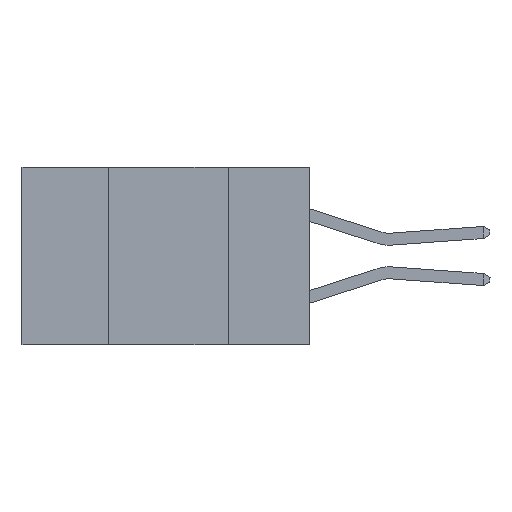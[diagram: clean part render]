
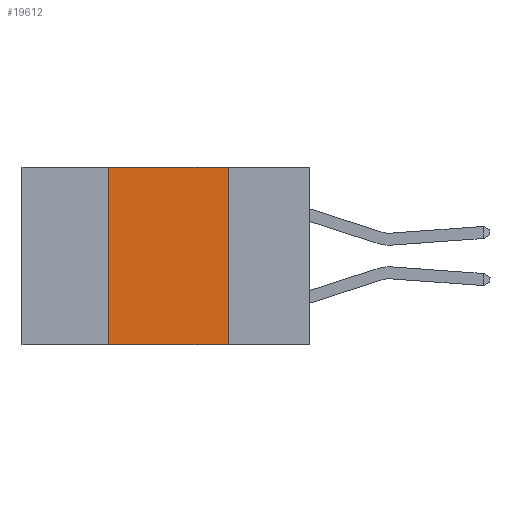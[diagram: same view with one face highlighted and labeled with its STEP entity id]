
A CAD part, left-side view. The second image highlights one B-rep face of the part: STEP entity #19612.
In plain terms, the highlighted planar face has unit normal (-1, 0, 0).
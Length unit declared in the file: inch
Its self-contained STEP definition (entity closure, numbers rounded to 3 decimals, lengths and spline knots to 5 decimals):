
#87 = EDGE_CURVE ( 'NONE', #4381, #3014, #8538, .T. ) ;
#420 = FACE_OUTER_BOUND ( 'NONE', #12172, .T. ) ;
#507 = CARTESIAN_POINT ( 'NONE',  ( 0., 0.42, 0. ) ) ;
#776 = LINE ( 'NONE', #15083, #2478 ) ;
#1242 = CARTESIAN_POINT ( 'NONE',  ( 0., 0.17, 0. ) ) ;
#1489 = CARTESIAN_POINT ( 'NONE',  ( 0., 0.6, 0. ) ) ;
#2449 = VERTEX_POINT ( 'NONE', #6908 ) ;
#2478 = VECTOR ( 'NONE', #12122, 39.37008 ) ;
#3014 = VERTEX_POINT ( 'NONE', #16948 ) ;
#3982 = LINE ( 'NONE', #1489, #16710 ) ;
#4381 = VERTEX_POINT ( 'NONE', #1242 ) ;
#5292 = DIRECTION ( 'NONE',  ( 0., 0., -1. ) ) ;
#5476 = VECTOR ( 'NONE', #8104, 39.37008 ) ;
#5951 = LINE ( 'NONE', #507, #5476 ) ;
#6462 = DIRECTION ( 'NONE',  ( 0., 0., -1. ) ) ;
#6529 = CARTESIAN_POINT ( 'NONE',  ( 0., 0.17, 0. ) ) ;
#6908 = CARTESIAN_POINT ( 'NONE',  ( 0., 0.42, 0. ) ) ;
#7217 = VERTEX_POINT ( 'NONE', #12631 ) ;
#7400 = EDGE_CURVE ( 'NONE', #7217, #3014, #776, .T. ) ;
#7825 = CARTESIAN_POINT ( 'NONE',  ( 0., 0.6, 0. ) ) ;
#8104 = DIRECTION ( 'NONE',  ( 0., 0., 1. ) ) ;
#8538 = LINE ( 'NONE', #6529, #12154 ) ;
#10066 = EDGE_CURVE ( 'NONE', #7217, #2449, #5951, .T. ) ;
#10313 = ORIENTED_EDGE ( 'NONE', *, *, #11594, .F. ) ;
#10852 = DIRECTION ( 'NONE',  ( 1., 0., 0. ) ) ;
#11594 = EDGE_CURVE ( 'NONE', #2449, #4381, #3982, .T. ) ;
#12122 = DIRECTION ( 'NONE',  ( 0., -1., 0. ) ) ;
#12154 = VECTOR ( 'NONE', #6462, 39.37008 ) ;
#12172 = EDGE_LOOP ( 'NONE', ( #15799, #10313, #19279, #12997 ) ) ;
#12631 = CARTESIAN_POINT ( 'NONE',  ( 0., 0.42, -0.37 ) ) ;
#12997 = ORIENTED_EDGE ( 'NONE', *, *, #7400, .T. ) ;
#15083 = CARTESIAN_POINT ( 'NONE',  ( 0., 0.6, -0.37 ) ) ;
#15495 = DIRECTION ( 'NONE',  ( 0., -1., 0. ) ) ;
#15799 = ORIENTED_EDGE ( 'NONE', *, *, #87, .F. ) ;
#16373 = AXIS2_PLACEMENT_3D ( 'NONE', #7825, #10852, #5292 ) ;
#16710 = VECTOR ( 'NONE', #15495, 39.37008 ) ;
#16944 = PLANE ( 'NONE',  #16373 ) ;
#16948 = CARTESIAN_POINT ( 'NONE',  ( 0., 0.17, -0.37 ) ) ;
#19279 = ORIENTED_EDGE ( 'NONE', *, *, #10066, .F. ) ;
#19612 = ADVANCED_FACE ( 'NONE', ( #420 ), #16944, .F. ) ;
